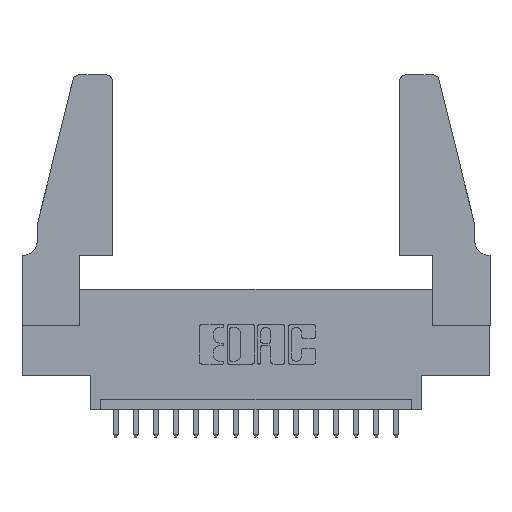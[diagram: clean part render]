
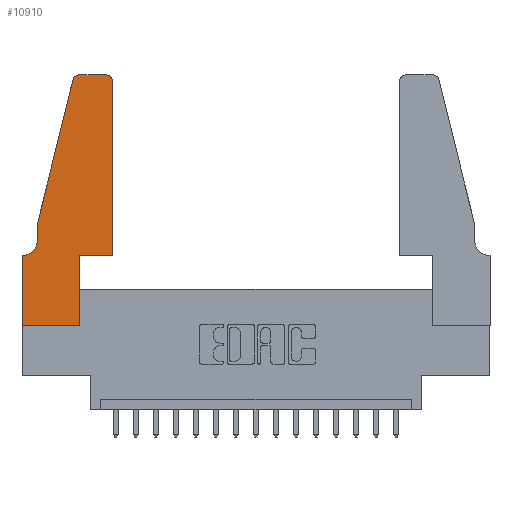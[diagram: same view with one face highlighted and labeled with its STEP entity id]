
A CAD part, top view. The second image highlights one B-rep face of the part: STEP entity #10910.
In plain terms, the highlighted planar face has unit normal (0, 0, 1).
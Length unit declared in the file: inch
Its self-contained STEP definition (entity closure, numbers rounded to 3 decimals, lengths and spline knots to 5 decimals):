
#239 = PLANE ( 'NONE',  #2116 ) ;
#265 = VERTEX_POINT ( 'NONE', #7332 ) ;
#280 = DIRECTION ( 'NONE',  ( 1., 0., 0. ) ) ;
#415 = ORIENTED_EDGE ( 'NONE', *, *, #15035, .T. ) ;
#656 = EDGE_CURVE ( 'NONE', #4421, #4773, #16556, .T. ) ;
#694 = VECTOR ( 'NONE', #6894, 39.37008 ) ;
#853 = CARTESIAN_POINT ( 'NONE',  ( 0.4505, 1.22, 0.37 ) ) ;
#872 = ORIENTED_EDGE ( 'NONE', *, *, #6158, .T. ) ;
#930 = EDGE_CURVE ( 'NONE', #9627, #16112, #9462, .T. ) ;
#1312 = DIRECTION ( 'NONE',  ( -0.239, -0.971, 0. ) ) ;
#1431 = LINE ( 'NONE', #15535, #16186 ) ;
#1983 = LINE ( 'NONE', #10376, #14254 ) ;
#2116 = AXIS2_PLACEMENT_3D ( 'NONE', #5589, #9363, #10710 ) ;
#2271 = DIRECTION ( 'NONE',  ( 1., 0., 0. ) ) ;
#2816 = CIRCLE ( 'NONE', #10773, 0.07 ) ;
#2913 = CARTESIAN_POINT ( 'NONE',  ( 0.284, 1.22, 0.37 ) ) ;
#3219 = DIRECTION ( 'NONE',  ( 1., 0., 0. ) ) ;
#3274 = AXIS2_PLACEMENT_3D ( 'NONE', #2913, #15018, #3219 ) ;
#4117 = VERTEX_POINT ( 'NONE', #7307 ) ;
#4190 = CARTESIAN_POINT ( 'NONE',  ( 0.0755, 0.5, 0.37 ) ) ;
#4303 = CARTESIAN_POINT ( 'NONE',  ( 0.0055, 0.42, 0.37 ) ) ;
#4421 = VERTEX_POINT ( 'NONE', #17205 ) ;
#4497 = VECTOR ( 'NONE', #10377, 39.37008 ) ;
#4710 = VECTOR ( 'NONE', #11464, 39.37008 ) ;
#4773 = VERTEX_POINT ( 'NONE', #14481 ) ;
#5201 = VECTOR ( 'NONE', #10356, 39.37008 ) ;
#5235 = CARTESIAN_POINT ( 'NONE',  ( 0., 0., 0.37 ) ) ;
#5589 = CARTESIAN_POINT ( 'NONE',  ( 0., 0.35, 0.37 ) ) ;
#5636 = DIRECTION ( 'NONE',  ( -1., 0., 0. ) ) ;
#5701 = EDGE_CURVE ( 'NONE', #4773, #9627, #1983, .T. ) ;
#5909 = CARTESIAN_POINT ( 'NONE',  ( 0.0755, 0.5, 0.37 ) ) ;
#6158 = EDGE_CURVE ( 'NONE', #265, #13764, #8839, .T. ) ;
#6355 = VECTOR ( 'NONE', #280, 39.37008 ) ;
#6439 = VERTEX_POINT ( 'NONE', #7193 ) ;
#6503 = ORIENTED_EDGE ( 'NONE', *, *, #16020, .T. ) ;
#6783 = ORIENTED_EDGE ( 'NONE', *, *, #16811, .T. ) ;
#6894 = DIRECTION ( 'NONE',  ( 0., -1., 0. ) ) ;
#7193 = CARTESIAN_POINT ( 'NONE',  ( 0., 0.35, 0.37 ) ) ;
#7307 = CARTESIAN_POINT ( 'NONE',  ( 0., 0., 0.37 ) ) ;
#7332 = CARTESIAN_POINT ( 'NONE',  ( 0.25487, 1.22718, 0.37 ) ) ;
#7373 = EDGE_CURVE ( 'NONE', #13764, #9710, #14191, .T. ) ;
#7816 = VECTOR ( 'NONE', #1312, 39.37008 ) ;
#8839 = LINE ( 'NONE', #8878, #7816 ) ;
#8878 = CARTESIAN_POINT ( 'NONE',  ( 0.0755, 0.5, 0.37 ) ) ;
#9075 = LINE ( 'NONE', #12550, #4710 ) ;
#9363 = DIRECTION ( 'NONE',  ( 0., 0., 1. ) ) ;
#9413 = EDGE_CURVE ( 'NONE', #4117, #13822, #12246, .T. ) ;
#9462 = CIRCLE ( 'NONE', #9484, 0.03 ) ;
#9471 = CARTESIAN_POINT ( 'NONE',  ( 0.4505, 0.35, 0.37 ) ) ;
#9484 = AXIS2_PLACEMENT_3D ( 'NONE', #13061, #10370, #2271 ) ;
#9627 = VERTEX_POINT ( 'NONE', #853 ) ;
#9710 = VERTEX_POINT ( 'NONE', #15026 ) ;
#10038 = ORIENTED_EDGE ( 'NONE', *, *, #13631, .T. ) ;
#10356 = DIRECTION ( 'NONE',  ( 1., 0., 0. ) ) ;
#10370 = DIRECTION ( 'NONE',  ( 0., 0., 1. ) ) ;
#10376 = CARTESIAN_POINT ( 'NONE',  ( 0.4505, 0.35, 0.37 ) ) ;
#10377 = DIRECTION ( 'NONE',  ( -1., 0., 0. ) ) ;
#10477 = ORIENTED_EDGE ( 'NONE', *, *, #16257, .T. ) ;
#10480 = VERTEX_POINT ( 'NONE', #12912 ) ;
#10538 = LINE ( 'NONE', #16803, #15328 ) ;
#10561 = ORIENTED_EDGE ( 'NONE', *, *, #5701, .T. ) ;
#10710 = DIRECTION ( 'NONE',  ( 1., 0., 0. ) ) ;
#10773 = AXIS2_PLACEMENT_3D ( 'NONE', #4303, #13588, #5636 ) ;
#10910 = ADVANCED_FACE ( 'NONE', ( #13455 ), #239, .T. ) ;
#11322 = CARTESIAN_POINT ( 'NONE',  ( 0.4205, 1.25, 0.37 ) ) ;
#11464 = DIRECTION ( 'NONE',  ( 0., 1., 0. ) ) ;
#11750 = CARTESIAN_POINT ( 'NONE',  ( 0.284, 1.25, 0.37 ) ) ;
#11862 = CARTESIAN_POINT ( 'NONE',  ( 0.2605, 1.25, 0.37 ) ) ;
#12246 = LINE ( 'NONE', #5235, #5201 ) ;
#12550 = CARTESIAN_POINT ( 'NONE',  ( 0.2865, 0.35, 0.37 ) ) ;
#12715 = EDGE_LOOP ( 'NONE', ( #6783, #10038, #872, #14303, #6503, #10477, #415, #15473, #17058, #16742, #10561, #16324 ) ) ;
#12851 = DIRECTION ( 'NONE',  ( 0., 1., 0. ) ) ;
#12912 = CARTESIAN_POINT ( 'NONE',  ( 0.0055, 0.35, 0.37 ) ) ;
#13061 = CARTESIAN_POINT ( 'NONE',  ( 0.4205, 1.22, 0.37 ) ) ;
#13455 = FACE_OUTER_BOUND ( 'NONE', #12715, .T. ) ;
#13588 = DIRECTION ( 'NONE',  ( 0., 0., -1. ) ) ;
#13631 = EDGE_CURVE ( 'NONE', #15159, #265, #13971, .T. ) ;
#13764 = VERTEX_POINT ( 'NONE', #5909 ) ;
#13822 = VERTEX_POINT ( 'NONE', #17015 ) ;
#13971 = CIRCLE ( 'NONE', #3274, 0.03 ) ;
#14168 = DIRECTION ( 'NONE',  ( -1., 0., 0. ) ) ;
#14191 = LINE ( 'NONE', #4190, #694 ) ;
#14254 = VECTOR ( 'NONE', #12851, 39.37008 ) ;
#14303 = ORIENTED_EDGE ( 'NONE', *, *, #7373, .T. ) ;
#14367 = DIRECTION ( 'NONE',  ( 0., -1., 0. ) ) ;
#14481 = CARTESIAN_POINT ( 'NONE',  ( 0.4505, 0.35, 0.37 ) ) ;
#15018 = DIRECTION ( 'NONE',  ( 0., 0., 1. ) ) ;
#15026 = CARTESIAN_POINT ( 'NONE',  ( 0.0755, 0.42, 0.37 ) ) ;
#15035 = EDGE_CURVE ( 'NONE', #6439, #4117, #1431, .T. ) ;
#15159 = VERTEX_POINT ( 'NONE', #11750 ) ;
#15328 = VECTOR ( 'NONE', #14168, 39.37008 ) ;
#15473 = ORIENTED_EDGE ( 'NONE', *, *, #9413, .T. ) ;
#15535 = CARTESIAN_POINT ( 'NONE',  ( 0., 0., 0.37 ) ) ;
#16020 = EDGE_CURVE ( 'NONE', #9710, #10480, #2816, .T. ) ;
#16112 = VERTEX_POINT ( 'NONE', #11322 ) ;
#16186 = VECTOR ( 'NONE', #14367, 39.37008 ) ;
#16257 = EDGE_CURVE ( 'NONE', #10480, #6439, #10538, .T. ) ;
#16324 = ORIENTED_EDGE ( 'NONE', *, *, #930, .T. ) ;
#16338 = LINE ( 'NONE', #11862, #4497 ) ;
#16556 = LINE ( 'NONE', #9471, #6355 ) ;
#16742 = ORIENTED_EDGE ( 'NONE', *, *, #656, .T. ) ;
#16803 = CARTESIAN_POINT ( 'NONE',  ( 0.0755, 0.35, 0.37 ) ) ;
#16811 = EDGE_CURVE ( 'NONE', #16112, #15159, #16338, .T. ) ;
#17015 = CARTESIAN_POINT ( 'NONE',  ( 0.2865, 0., 0.37 ) ) ;
#17058 = ORIENTED_EDGE ( 'NONE', *, *, #17212, .T. ) ;
#17205 = CARTESIAN_POINT ( 'NONE',  ( 0.2865, 0.35, 0.37 ) ) ;
#17212 = EDGE_CURVE ( 'NONE', #13822, #4421, #9075, .T. ) ;
